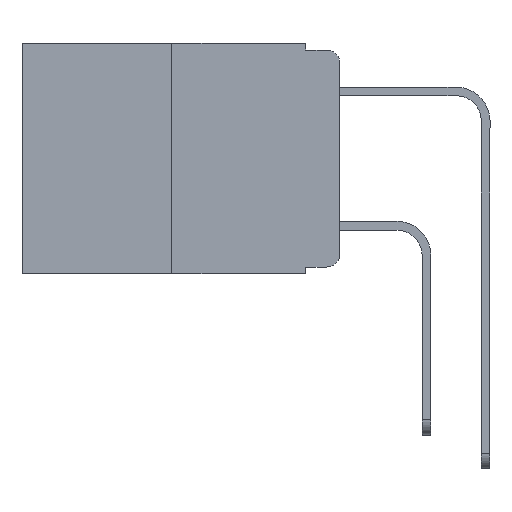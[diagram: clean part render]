
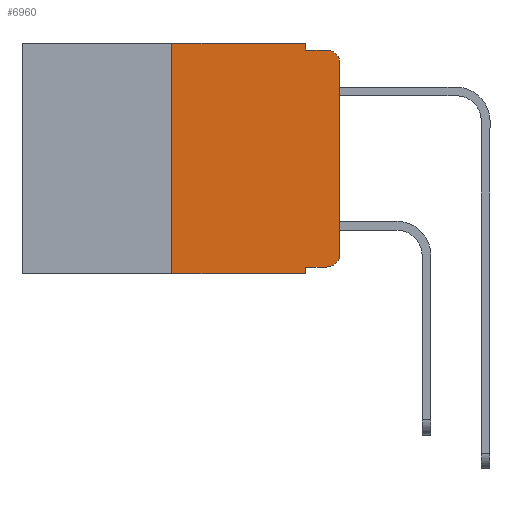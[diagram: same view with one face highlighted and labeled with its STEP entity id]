
A CAD part, left-side view. The second image highlights one B-rep face of the part: STEP entity #6960.
In plain terms, the highlighted planar face has unit normal (-1, 0, 0).
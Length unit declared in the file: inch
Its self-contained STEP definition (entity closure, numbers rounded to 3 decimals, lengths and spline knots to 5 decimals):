
#36 = VERTEX_POINT ( 'NONE', #10107 ) ;
#121 = AXIS2_PLACEMENT_3D ( 'NONE', #8434, #1218, #9615 ) ;
#172 = EDGE_CURVE ( 'NONE', #9569, #10845, #9070, .T. ) ;
#452 = ORIENTED_EDGE ( 'NONE', *, *, #5254, .F. ) ;
#459 = CARTESIAN_POINT ( 'NONE',  ( 0., 0.051, -0.01 ) ) ;
#656 = CARTESIAN_POINT ( 'NONE',  ( 0., 0.051, 0. ) ) ;
#712 = DIRECTION ( 'NONE',  ( 0., 0., -1. ) ) ;
#898 = ORIENTED_EDGE ( 'NONE', *, *, #11751, .F. ) ;
#1035 = CARTESIAN_POINT ( 'NONE',  ( 0., 0., 0. ) ) ;
#1066 = LINE ( 'NONE', #12469, #11049 ) ;
#1096 = EDGE_CURVE ( 'NONE', #36, #9569, #13791, .T. ) ;
#1218 = DIRECTION ( 'NONE',  ( 1., 0., 0. ) ) ;
#1251 = VERTEX_POINT ( 'NONE', #1470 ) ;
#1470 = CARTESIAN_POINT ( 'NONE',  ( 0., 0.02, -0.01 ) ) ;
#1551 = CARTESIAN_POINT ( 'NONE',  ( 0., 0.02, -0.03 ) ) ;
#1704 = ORIENTED_EDGE ( 'NONE', *, *, #1096, .T. ) ;
#1963 = EDGE_CURVE ( 'NONE', #36, #6590, #8972, .T. ) ;
#2108 = ORIENTED_EDGE ( 'NONE', *, *, #172, .T. ) ;
#2741 = CARTESIAN_POINT ( 'NONE',  ( 0., 0.02, -0.313 ) ) ;
#2802 = EDGE_CURVE ( 'NONE', #13315, #11711, #8189, .T. ) ;
#2817 = DIRECTION ( 'NONE',  ( 0., 0., -1. ) ) ;
#2896 = CARTESIAN_POINT ( 'NONE',  ( 0., 0., -0.313 ) ) ;
#3317 = VERTEX_POINT ( 'NONE', #459 ) ;
#3331 = CARTESIAN_POINT ( 'NONE',  ( 0., 0.473, -0.343 ) ) ;
#3848 = ORIENTED_EDGE ( 'NONE', *, *, #4445, .F. ) ;
#4163 = DIRECTION ( 'NONE',  ( 0., -1., 0. ) ) ;
#4225 = ORIENTED_EDGE ( 'NONE', *, *, #2802, .F. ) ;
#4445 = EDGE_CURVE ( 'NONE', #4756, #3317, #14842, .T. ) ;
#4478 = DIRECTION ( 'NONE',  ( 0., -1., 0. ) ) ;
#4740 = CARTESIAN_POINT ( 'NONE',  ( 0., 0.02, -0.333 ) ) ;
#4756 = VERTEX_POINT ( 'NONE', #6708 ) ;
#5038 = CARTESIAN_POINT ( 'NONE',  ( 0., 0.051, 0. ) ) ;
#5254 = EDGE_CURVE ( 'NONE', #3317, #1251, #13978, .T. ) ;
#5378 = VECTOR ( 'NONE', #9452, 39.37008 ) ;
#5423 = VECTOR ( 'NONE', #11857, 39.37008 ) ;
#6056 = EDGE_CURVE ( 'NONE', #9130, #1251, #12318, .T. ) ;
#6122 = LINE ( 'NONE', #1035, #5378 ) ;
#6226 = CARTESIAN_POINT ( 'NONE',  ( 0., 0.051, -0.01 ) ) ;
#6242 = LINE ( 'NONE', #3331, #14732 ) ;
#6251 = CARTESIAN_POINT ( 'NONE',  ( 0., 0.051, -0.333 ) ) ;
#6590 = VERTEX_POINT ( 'NONE', #8865 ) ;
#6672 = FACE_OUTER_BOUND ( 'NONE', #9078, .T. ) ;
#6708 = CARTESIAN_POINT ( 'NONE',  ( 0., 0.051, 0. ) ) ;
#6960 = ADVANCED_FACE ( 'NONE', ( #6672 ), #8381, .F. ) ;
#7482 = CARTESIAN_POINT ( 'NONE',  ( 0., 0.25, -0.343 ) ) ;
#8189 = LINE ( 'NONE', #11173, #10149 ) ;
#8369 = EDGE_CURVE ( 'NONE', #10845, #9130, #6122, .T. ) ;
#8381 = PLANE ( 'NONE',  #121 ) ;
#8434 = CARTESIAN_POINT ( 'NONE',  ( 0., 0.473, 0. ) ) ;
#8546 = AXIS2_PLACEMENT_3D ( 'NONE', #2741, #9320, #9298 ) ;
#8865 = CARTESIAN_POINT ( 'NONE',  ( 0., 0.051, -0.343 ) ) ;
#8972 = LINE ( 'NONE', #656, #14052 ) ;
#9070 = CIRCLE ( 'NONE', #8546, 0.02 ) ;
#9078 = EDGE_LOOP ( 'NONE', ( #9394, #12620, #452, #3848, #898, #4225, #10418, #10749, #1704, #2108 ) ) ;
#9130 = VERTEX_POINT ( 'NONE', #9625 ) ;
#9298 = DIRECTION ( 'NONE',  ( 0., 0., -1. ) ) ;
#9320 = DIRECTION ( 'NONE',  ( -1., 0., 0. ) ) ;
#9394 = ORIENTED_EDGE ( 'NONE', *, *, #8369, .T. ) ;
#9452 = DIRECTION ( 'NONE',  ( 0., 0., 1. ) ) ;
#9569 = VERTEX_POINT ( 'NONE', #4740 ) ;
#9615 = DIRECTION ( 'NONE',  ( 0., 0., -1. ) ) ;
#9625 = CARTESIAN_POINT ( 'NONE',  ( 0., 0., -0.03 ) ) ;
#9887 = DIRECTION ( 'NONE',  ( -1., 0., 0. ) ) ;
#10107 = CARTESIAN_POINT ( 'NONE',  ( 0., 0.051, -0.333 ) ) ;
#10149 = VECTOR ( 'NONE', #11349, 39.37008 ) ;
#10418 = ORIENTED_EDGE ( 'NONE', *, *, #11099, .T. ) ;
#10749 = ORIENTED_EDGE ( 'NONE', *, *, #1963, .F. ) ;
#10845 = VERTEX_POINT ( 'NONE', #2896 ) ;
#10924 = VECTOR ( 'NONE', #4163, 39.37008 ) ;
#11049 = VECTOR ( 'NONE', #4478, 39.37008 ) ;
#11099 = EDGE_CURVE ( 'NONE', #13315, #6590, #6242, .T. ) ;
#11173 = CARTESIAN_POINT ( 'NONE',  ( 0., 0.25, 0. ) ) ;
#11349 = DIRECTION ( 'NONE',  ( 0., 0., 1. ) ) ;
#11688 = AXIS2_PLACEMENT_3D ( 'NONE', #1551, #9887, #2817 ) ;
#11711 = VERTEX_POINT ( 'NONE', #14536 ) ;
#11751 = EDGE_CURVE ( 'NONE', #11711, #4756, #1066, .T. ) ;
#11857 = DIRECTION ( 'NONE',  ( 0., -1., 0. ) ) ;
#12008 = VECTOR ( 'NONE', #12944, 39.37008 ) ;
#12318 = CIRCLE ( 'NONE', #11688, 0.02 ) ;
#12469 = CARTESIAN_POINT ( 'NONE',  ( 0., 0.473, 0. ) ) ;
#12620 = ORIENTED_EDGE ( 'NONE', *, *, #6056, .T. ) ;
#12944 = DIRECTION ( 'NONE',  ( 0., 0., -1. ) ) ;
#13315 = VERTEX_POINT ( 'NONE', #7482 ) ;
#13627 = DIRECTION ( 'NONE',  ( 0., -1., 0. ) ) ;
#13791 = LINE ( 'NONE', #6251, #10924 ) ;
#13978 = LINE ( 'NONE', #6226, #5423 ) ;
#14052 = VECTOR ( 'NONE', #712, 39.37008 ) ;
#14536 = CARTESIAN_POINT ( 'NONE',  ( 0., 0.25, 0. ) ) ;
#14732 = VECTOR ( 'NONE', #13627, 39.37008 ) ;
#14842 = LINE ( 'NONE', #5038, #12008 ) ;
